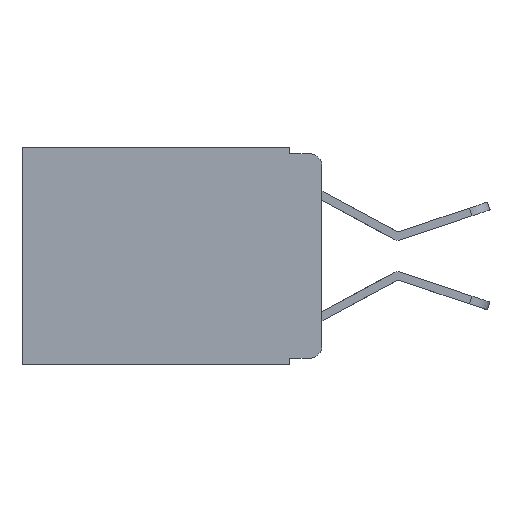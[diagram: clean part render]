
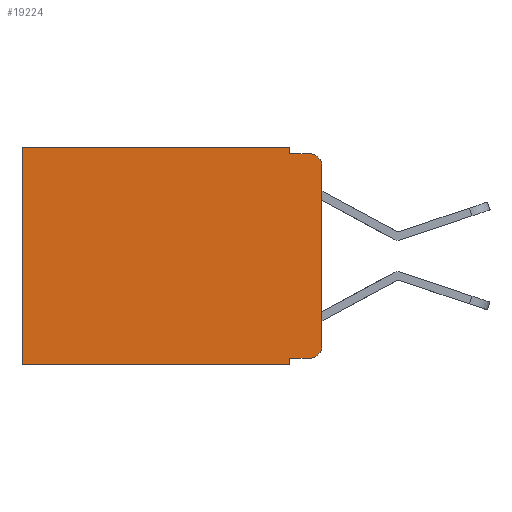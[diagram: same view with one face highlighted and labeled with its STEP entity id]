
A CAD part, left-side view. The second image highlights one B-rep face of the part: STEP entity #19224.
In plain terms, the highlighted planar face has unit normal (-1, 0, 0).
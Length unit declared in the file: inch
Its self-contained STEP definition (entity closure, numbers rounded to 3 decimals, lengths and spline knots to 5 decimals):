
#430 = ORIENTED_EDGE ( 'NONE', *, *, #20325, .T. ) ;
#584 = CIRCLE ( 'NONE', #8585, 0.02 ) ;
#764 = LINE ( 'NONE', #20757, #13775 ) ;
#935 = CARTESIAN_POINT ( 'NONE',  ( 0.298, 0., 0. ) ) ;
#1416 = DIRECTION ( 'NONE',  ( 1., 0., 0. ) ) ;
#1538 = VERTEX_POINT ( 'NONE', #14086 ) ;
#2637 = ORIENTED_EDGE ( 'NONE', *, *, #5919, .F. ) ;
#2731 = DIRECTION ( 'NONE',  ( 0., 0., -1. ) ) ;
#3118 = CARTESIAN_POINT ( 'NONE',  ( 0.298, 0.051, 0. ) ) ;
#3237 = CIRCLE ( 'NONE', #7255, 0.02 ) ;
#3307 = EDGE_LOOP ( 'NONE', ( #3554, #15113, #16059, #19606, #430, #15700, #14296, #2637, #15914, #11451 ) ) ;
#3493 = VERTEX_POINT ( 'NONE', #15370 ) ;
#3554 = ORIENTED_EDGE ( 'NONE', *, *, #5814, .F. ) ;
#3778 = DIRECTION ( 'NONE',  ( -1., 0., 0. ) ) ;
#3786 = CARTESIAN_POINT ( 'NONE',  ( 0.298, 0., -0.313 ) ) ;
#4032 = EDGE_CURVE ( 'NONE', #3493, #19805, #17746, .T. ) ;
#4351 = VERTEX_POINT ( 'NONE', #8544 ) ;
#5393 = VERTEX_POINT ( 'NONE', #11588 ) ;
#5814 = EDGE_CURVE ( 'NONE', #5393, #10216, #13023, .T. ) ;
#5919 = EDGE_CURVE ( 'NONE', #18517, #1538, #14311, .T. ) ;
#6033 = VECTOR ( 'NONE', #19301, 39.37008 ) ;
#6060 = VECTOR ( 'NONE', #17798, 39.37008 ) ;
#6632 = VECTOR ( 'NONE', #20668, 39.37008 ) ;
#6790 = VERTEX_POINT ( 'NONE', #7123 ) ;
#7123 = CARTESIAN_POINT ( 'NONE',  ( 0.298, 0.051, 0. ) ) ;
#7255 = AXIS2_PLACEMENT_3D ( 'NONE', #18642, #3778, #17057 ) ;
#7413 = CARTESIAN_POINT ( 'NONE',  ( 0.298, 0.02, -0.01 ) ) ;
#7800 = LINE ( 'NONE', #14107, #16857 ) ;
#8382 = CARTESIAN_POINT ( 'NONE',  ( 0.298, 0.473, -0.343 ) ) ;
#8544 = CARTESIAN_POINT ( 'NONE',  ( 0.298, 0.051, -0.01 ) ) ;
#8545 = CARTESIAN_POINT ( 'NONE',  ( 0.298, 0.051, -0.333 ) ) ;
#8585 = AXIS2_PLACEMENT_3D ( 'NONE', #17325, #9220, #15963 ) ;
#8628 = EDGE_CURVE ( 'NONE', #5393, #14508, #584, .T. ) ;
#9220 = DIRECTION ( 'NONE',  ( -1., 0., 0. ) ) ;
#9240 = DIRECTION ( 'NONE',  ( 0., 1., 0. ) ) ;
#9488 = EDGE_CURVE ( 'NONE', #18517, #14594, #17175, .T. ) ;
#9501 = VECTOR ( 'NONE', #13868, 39.37008 ) ;
#9715 = PLANE ( 'NONE',  #11217 ) ;
#9899 = VECTOR ( 'NONE', #11561, 39.37008 ) ;
#10216 = VERTEX_POINT ( 'NONE', #3786 ) ;
#10540 = CARTESIAN_POINT ( 'NONE',  ( 0.298, 0.051, 0. ) ) ;
#10977 = EDGE_CURVE ( 'NONE', #4351, #14508, #7800, .T. ) ;
#11095 = EDGE_CURVE ( 'NONE', #1538, #19805, #17122, .T. ) ;
#11140 = DIRECTION ( 'NONE',  ( 0., 1., 0. ) ) ;
#11217 = AXIS2_PLACEMENT_3D ( 'NONE', #16035, #1416, #2731 ) ;
#11362 = CARTESIAN_POINT ( 'NONE',  ( 0.298, 0.051, -0.333 ) ) ;
#11451 = ORIENTED_EDGE ( 'NONE', *, *, #13588, .T. ) ;
#11561 = DIRECTION ( 'NONE',  ( 0., 0., -1. ) ) ;
#11588 = CARTESIAN_POINT ( 'NONE',  ( 0.298, 0., -0.03 ) ) ;
#11990 = CARTESIAN_POINT ( 'NONE',  ( 0.298, 0.473, 0. ) ) ;
#13023 = LINE ( 'NONE', #935, #6033 ) ;
#13588 = EDGE_CURVE ( 'NONE', #14594, #10216, #3237, .T. ) ;
#13775 = VECTOR ( 'NONE', #9240, 39.37008 ) ;
#13868 = DIRECTION ( 'NONE',  ( 0., 0., -1. ) ) ;
#14073 = CARTESIAN_POINT ( 'NONE',  ( 0.298, 0.02, -0.333 ) ) ;
#14086 = CARTESIAN_POINT ( 'NONE',  ( 0.298, 0.051, -0.343 ) ) ;
#14107 = CARTESIAN_POINT ( 'NONE',  ( 0.298, 0.051, -0.01 ) ) ;
#14296 = ORIENTED_EDGE ( 'NONE', *, *, #11095, .F. ) ;
#14311 = LINE ( 'NONE', #3118, #9899 ) ;
#14508 = VERTEX_POINT ( 'NONE', #7413 ) ;
#14594 = VERTEX_POINT ( 'NONE', #14073 ) ;
#14757 = CARTESIAN_POINT ( 'NONE',  ( 0.298, 0., -0.343 ) ) ;
#14809 = VECTOR ( 'NONE', #11140, 39.37008 ) ;
#15113 = ORIENTED_EDGE ( 'NONE', *, *, #8628, .T. ) ;
#15370 = CARTESIAN_POINT ( 'NONE',  ( 0.298, 0.473, 0. ) ) ;
#15700 = ORIENTED_EDGE ( 'NONE', *, *, #4032, .T. ) ;
#15914 = ORIENTED_EDGE ( 'NONE', *, *, #9488, .T. ) ;
#15963 = DIRECTION ( 'NONE',  ( 0., 0., -1. ) ) ;
#16035 = CARTESIAN_POINT ( 'NONE',  ( 0.298, 0., 0. ) ) ;
#16059 = ORIENTED_EDGE ( 'NONE', *, *, #10977, .F. ) ;
#16653 = FACE_OUTER_BOUND ( 'NONE', #3307, .T. ) ;
#16857 = VECTOR ( 'NONE', #19305, 39.37008 ) ;
#17057 = DIRECTION ( 'NONE',  ( 0., 0., -1. ) ) ;
#17122 = LINE ( 'NONE', #14757, #14809 ) ;
#17175 = LINE ( 'NONE', #11362, #6060 ) ;
#17264 = LINE ( 'NONE', #10540, #9501 ) ;
#17325 = CARTESIAN_POINT ( 'NONE',  ( 0.298, 0.02, -0.03 ) ) ;
#17491 = EDGE_CURVE ( 'NONE', #6790, #4351, #17264, .T. ) ;
#17746 = LINE ( 'NONE', #11990, #6632 ) ;
#17798 = DIRECTION ( 'NONE',  ( 0., -1., 0. ) ) ;
#18517 = VERTEX_POINT ( 'NONE', #8545 ) ;
#18642 = CARTESIAN_POINT ( 'NONE',  ( 0.298, 0.02, -0.313 ) ) ;
#19224 = ADVANCED_FACE ( 'NONE', ( #16653 ), #9715, .F. ) ;
#19301 = DIRECTION ( 'NONE',  ( 0., 0., -1. ) ) ;
#19305 = DIRECTION ( 'NONE',  ( 0., -1., 0. ) ) ;
#19606 = ORIENTED_EDGE ( 'NONE', *, *, #17491, .F. ) ;
#19805 = VERTEX_POINT ( 'NONE', #8382 ) ;
#20325 = EDGE_CURVE ( 'NONE', #6790, #3493, #764, .T. ) ;
#20668 = DIRECTION ( 'NONE',  ( 0., 0., -1. ) ) ;
#20757 = CARTESIAN_POINT ( 'NONE',  ( 0.298, 0., 0. ) ) ;
